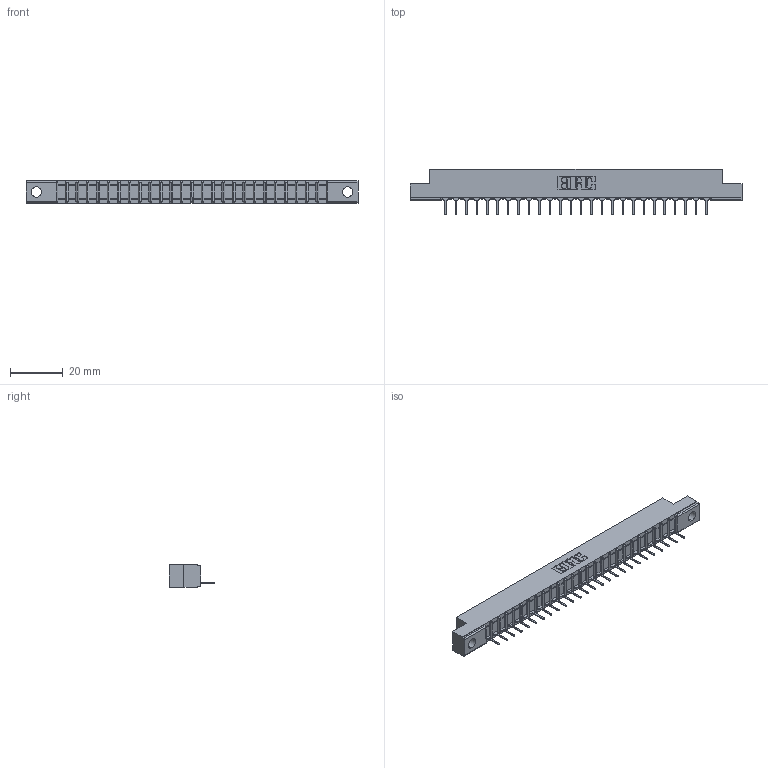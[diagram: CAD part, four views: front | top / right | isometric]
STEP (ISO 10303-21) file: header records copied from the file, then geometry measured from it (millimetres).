
FILE_DESCRIPTION (( 'STEP AP203' ), '1' );
FILE_NAME ('307-026-531-104.STEP', '2019-09-03T21:48:07', ( '' ), ( '' ), 'SwSTEP 2.0', 'SolidWorks 2016', '' );
FILE_SCHEMA (( 'CONFIG_CONTROL_DESIGN' ));
Length unit declared in the file: inch
Products named in the file (3): 307 Part_.156 Dia Mounting Holes; 307-026-531-104; 307-290-001_531
Assembly tree (27 placements, depth 2):
  307-026-531-104
    307 Part_.156 Dia Mounting Holes
    307-290-001_531  x26
Bounding box: 126.03 x 17.42 x 8.71 mm (x, y, z)
Volume: 7793.8 mm3; surface area: 11838.2 mm2
Topology: 27 solids, 27 shells, 1615 faces, 4571 edges, 2938 vertices
Faces by surface type: plane 1046, cylinder 515, sphere 54
Entity records: 24648 total; most frequent: CARTESIAN_POINT 4150, ORIENTED_EDGE 4134, DIRECTION 4037, EDGE_CURVE 2067, VECTOR 1587, LINE 1587, VERTEX_POINT 1338, AXIS2_PLACEMENT_3D 1225
